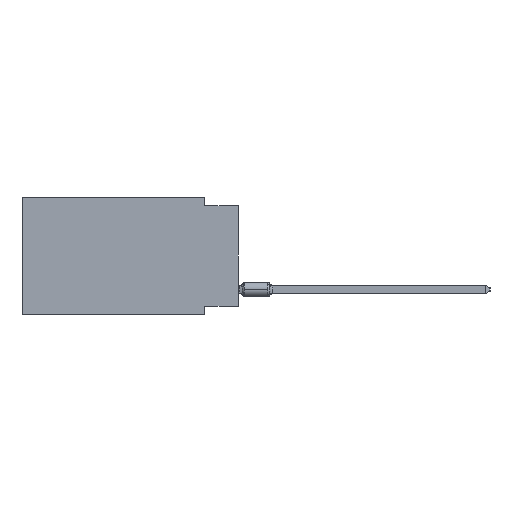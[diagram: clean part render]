
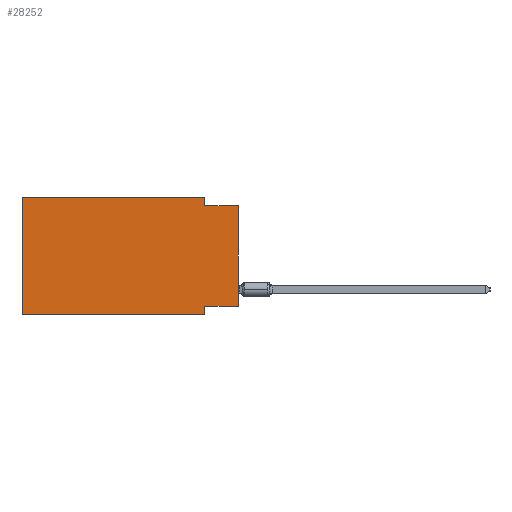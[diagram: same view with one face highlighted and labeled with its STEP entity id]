
A CAD part, left-side view. The second image highlights one B-rep face of the part: STEP entity #28252.
In plain terms, the highlighted planar face has unit normal (-1, 0, 0).
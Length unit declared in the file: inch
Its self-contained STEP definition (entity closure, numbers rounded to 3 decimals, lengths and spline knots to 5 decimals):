
#568 = CARTESIAN_POINT ( 'NONE',  ( 0., 0.1, -0.35 ) ) ;
#780 = CARTESIAN_POINT ( 'NONE',  ( 0., 0.1, -0.325 ) ) ;
#904 = VECTOR ( 'NONE', #1628, 39.37008 ) ;
#1267 = EDGE_CURVE ( 'NONE', #36853, #41313, #39352, .T. ) ;
#1628 = DIRECTION ( 'NONE',  ( 0., 0., 1. ) ) ;
#2397 = EDGE_CURVE ( 'NONE', #23988, #41313, #33305, .T. ) ;
#2732 = DIRECTION ( 'NONE',  ( 0., -1., 0. ) ) ;
#5007 = DIRECTION ( 'NONE',  ( 0., 1., 0. ) ) ;
#6698 = ORIENTED_EDGE ( 'NONE', *, *, #1267, .F. ) ;
#7313 = CARTESIAN_POINT ( 'NONE',  ( 0., 0., 0. ) ) ;
#7324 = DIRECTION ( 'NONE',  ( 0., -1., 0. ) ) ;
#7494 = VECTOR ( 'NONE', #7324, 39.37008 ) ;
#7701 = VECTOR ( 'NONE', #31099, 39.37008 ) ;
#7911 = CARTESIAN_POINT ( 'NONE',  ( 0., 0.1, 0. ) ) ;
#7974 = EDGE_CURVE ( 'NONE', #23988, #21623, #24968, .T. ) ;
#8126 = PLANE ( 'NONE',  #31387 ) ;
#9910 = DIRECTION ( 'NONE',  ( 0., 0., -1. ) ) ;
#9916 = CARTESIAN_POINT ( 'NONE',  ( 0., 0.645, -0.35 ) ) ;
#10190 = ORIENTED_EDGE ( 'NONE', *, *, #23633, .F. ) ;
#11546 = ORIENTED_EDGE ( 'NONE', *, *, #7974, .F. ) ;
#12389 = CARTESIAN_POINT ( 'NONE',  ( 0., 0.645, 0. ) ) ;
#13892 = CARTESIAN_POINT ( 'NONE',  ( 0., 0.645, -0.35 ) ) ;
#13993 = CARTESIAN_POINT ( 'NONE',  ( 0., 0.645, 0. ) ) ;
#14440 = VERTEX_POINT ( 'NONE', #35985 ) ;
#15349 = LINE ( 'NONE', #32643, #21177 ) ;
#15711 = DIRECTION ( 'NONE',  ( 0., 0., -1. ) ) ;
#17170 = VECTOR ( 'NONE', #5007, 39.37008 ) ;
#18049 = DIRECTION ( 'NONE',  ( 0., 0., 1. ) ) ;
#18357 = VECTOR ( 'NONE', #9910, 39.37008 ) ;
#18716 = VERTEX_POINT ( 'NONE', #23844 ) ;
#19264 = ORIENTED_EDGE ( 'NONE', *, *, #32156, .F. ) ;
#20494 = ORIENTED_EDGE ( 'NONE', *, *, #22934, .F. ) ;
#21177 = VECTOR ( 'NONE', #2732, 39.37008 ) ;
#21229 = EDGE_CURVE ( 'NONE', #32654, #26880, #31117, .T. ) ;
#21623 = VERTEX_POINT ( 'NONE', #13993 ) ;
#21911 = LINE ( 'NONE', #35141, #17170 ) ;
#22191 = DIRECTION ( 'NONE',  ( 1., 0., 0. ) ) ;
#22934 = EDGE_CURVE ( 'NONE', #32654, #36853, #21911, .T. ) ;
#23119 = DIRECTION ( 'NONE',  ( 0., -1., 0. ) ) ;
#23283 = VECTOR ( 'NONE', #23119, 39.37008 ) ;
#23633 = EDGE_CURVE ( 'NONE', #21623, #18716, #33754, .T. ) ;
#23791 = CARTESIAN_POINT ( 'NONE',  ( 0., 0.645, 0. ) ) ;
#23844 = CARTESIAN_POINT ( 'NONE',  ( 0., 0.1, 0. ) ) ;
#23988 = VERTEX_POINT ( 'NONE', #13892 ) ;
#24684 = CARTESIAN_POINT ( 'NONE',  ( 0., 0.1, -0.35 ) ) ;
#24968 = LINE ( 'NONE', #12389, #25234 ) ;
#25234 = VECTOR ( 'NONE', #18049, 39.37008 ) ;
#26557 = EDGE_LOOP ( 'NONE', ( #32492, #19264, #30425, #10190, #11546, #26782, #6698, #20494 ) ) ;
#26782 = ORIENTED_EDGE ( 'NONE', *, *, #2397, .T. ) ;
#26880 = VERTEX_POINT ( 'NONE', #33788 ) ;
#28252 = ADVANCED_FACE ( 'NONE', ( #41915 ), #8126, .F. ) ;
#30425 = ORIENTED_EDGE ( 'NONE', *, *, #38692, .F. ) ;
#31099 = DIRECTION ( 'NONE',  ( 0., 0., -1. ) ) ;
#31117 = LINE ( 'NONE', #7313, #904 ) ;
#31387 = AXIS2_PLACEMENT_3D ( 'NONE', #31945, #22191, #15711 ) ;
#31945 = CARTESIAN_POINT ( 'NONE',  ( 0., 0.645, 0. ) ) ;
#32156 = EDGE_CURVE ( 'NONE', #14440, #26880, #15349, .T. ) ;
#32492 = ORIENTED_EDGE ( 'NONE', *, *, #21229, .T. ) ;
#32643 = CARTESIAN_POINT ( 'NONE',  ( 0., 0., -0.025 ) ) ;
#32654 = VERTEX_POINT ( 'NONE', #42789 ) ;
#33305 = LINE ( 'NONE', #9916, #23283 ) ;
#33754 = LINE ( 'NONE', #23791, #7494 ) ;
#33788 = CARTESIAN_POINT ( 'NONE',  ( 0., 0., -0.025 ) ) ;
#35141 = CARTESIAN_POINT ( 'NONE',  ( 0., 0., -0.325 ) ) ;
#35985 = CARTESIAN_POINT ( 'NONE',  ( 0., 0.1, -0.025 ) ) ;
#36853 = VERTEX_POINT ( 'NONE', #780 ) ;
#37600 = LINE ( 'NONE', #7911, #7701 ) ;
#38692 = EDGE_CURVE ( 'NONE', #18716, #14440, #37600, .T. ) ;
#39352 = LINE ( 'NONE', #568, #18357 ) ;
#41313 = VERTEX_POINT ( 'NONE', #24684 ) ;
#41915 = FACE_OUTER_BOUND ( 'NONE', #26557, .T. ) ;
#42789 = CARTESIAN_POINT ( 'NONE',  ( 0., 0., -0.325 ) ) ;
